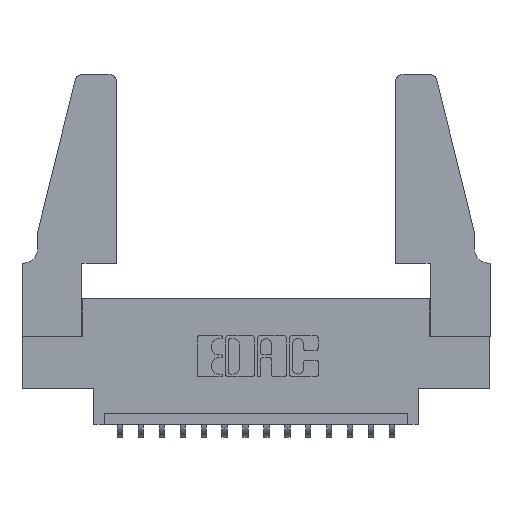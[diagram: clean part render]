
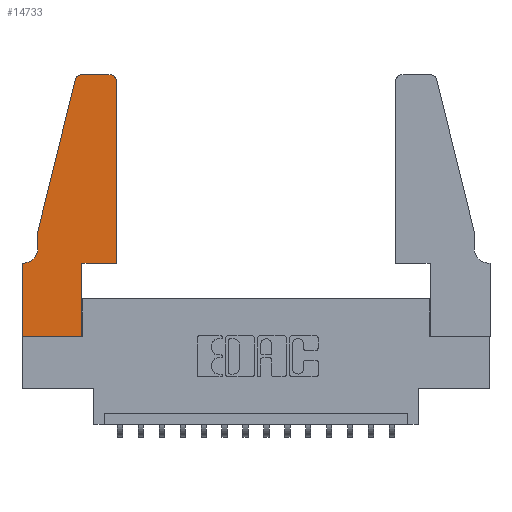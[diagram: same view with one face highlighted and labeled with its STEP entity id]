
A CAD part, top view. The second image highlights one B-rep face of the part: STEP entity #14733.
In plain terms, the highlighted planar face has unit normal (0, 0, 1).
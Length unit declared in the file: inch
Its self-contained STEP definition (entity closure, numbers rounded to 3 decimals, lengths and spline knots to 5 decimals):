
#76 = DIRECTION ( 'NONE',  ( 1., 0., 0. ) ) ;
#94 = CARTESIAN_POINT ( 'NONE',  ( 0.284, 1.25, 0.37 ) ) ;
#115 = AXIS2_PLACEMENT_3D ( 'NONE', #10868, #9346, #8216 ) ;
#148 = DIRECTION ( 'NONE',  ( 1., 0., 0. ) ) ;
#444 = VECTOR ( 'NONE', #148, 39.37008 ) ;
#656 = VECTOR ( 'NONE', #3718, 39.37008 ) ;
#695 = PLANE ( 'NONE',  #3113 ) ;
#698 = LINE ( 'NONE', #9634, #4725 ) ;
#718 = DIRECTION ( 'NONE',  ( 0., -1., 0. ) ) ;
#967 = AXIS2_PLACEMENT_3D ( 'NONE', #3220, #9567, #7124 ) ;
#976 = LINE ( 'NONE', #12297, #14297 ) ;
#1008 = VERTEX_POINT ( 'NONE', #6383 ) ;
#1136 = EDGE_LOOP ( 'NONE', ( #13993, #15913, #9920, #2115, #15725, #8309, #8147, #14769, #15879, #13197, #11582, #14621 ) ) ;
#1355 = DIRECTION ( 'NONE',  ( 0., 0., 1. ) ) ;
#1687 = LINE ( 'NONE', #6221, #16185 ) ;
#1898 = CIRCLE ( 'NONE', #967, 0.03 ) ;
#2115 = ORIENTED_EDGE ( 'NONE', *, *, #6302, .T. ) ;
#2418 = DIRECTION ( 'NONE',  ( 0., -1., 0. ) ) ;
#2438 = CARTESIAN_POINT ( 'NONE',  ( 0.0755, 0.35, 0.37 ) ) ;
#3079 = LINE ( 'NONE', #16092, #9703 ) ;
#3113 = AXIS2_PLACEMENT_3D ( 'NONE', #16163, #10983, #14784 ) ;
#3220 = CARTESIAN_POINT ( 'NONE',  ( 0.4205, 1.22, 0.37 ) ) ;
#3603 = VERTEX_POINT ( 'NONE', #14075 ) ;
#3718 = DIRECTION ( 'NONE',  ( 0., 1., 0. ) ) ;
#4295 = DIRECTION ( 'NONE',  ( 1., 0., 0. ) ) ;
#4384 = EDGE_CURVE ( 'NONE', #14108, #9184, #15170, .T. ) ;
#4507 = CARTESIAN_POINT ( 'NONE',  ( 0.0755, 0.5, 0.37 ) ) ;
#4725 = VECTOR ( 'NONE', #4295, 39.37008 ) ;
#4752 = CARTESIAN_POINT ( 'NONE',  ( 0.0755, 0.5, 0.37 ) ) ;
#4783 = DIRECTION ( 'NONE',  ( -1., 0., 0. ) ) ;
#4927 = CARTESIAN_POINT ( 'NONE',  ( 0.4205, 1.25, 0.37 ) ) ;
#5158 = DIRECTION ( 'NONE',  ( 0., 1., 0. ) ) ;
#5824 = CIRCLE ( 'NONE', #13679, 0.03 ) ;
#6013 = EDGE_CURVE ( 'NONE', #10647, #8459, #5824, .T. ) ;
#6221 = CARTESIAN_POINT ( 'NONE',  ( 0.4505, 0.35, 0.37 ) ) ;
#6302 = EDGE_CURVE ( 'NONE', #6446, #16093, #976, .T. ) ;
#6353 = CARTESIAN_POINT ( 'NONE',  ( 0.2605, 1.25, 0.37 ) ) ;
#6383 = CARTESIAN_POINT ( 'NONE',  ( 0.4505, 1.22, 0.37 ) ) ;
#6446 = VERTEX_POINT ( 'NONE', #4507 ) ;
#7049 = CIRCLE ( 'NONE', #115, 0.07 ) ;
#7124 = DIRECTION ( 'NONE',  ( 1., 0., 0. ) ) ;
#7454 = LINE ( 'NONE', #15557, #444 ) ;
#7640 = DIRECTION ( 'NONE',  ( -1., 0., 0. ) ) ;
#7692 = LINE ( 'NONE', #4752, #7885 ) ;
#7705 = CARTESIAN_POINT ( 'NONE',  ( 0.284, 1.22, 0.37 ) ) ;
#7885 = VECTOR ( 'NONE', #9975, 39.37008 ) ;
#8147 = ORIENTED_EDGE ( 'NONE', *, *, #14556, .T. ) ;
#8216 = DIRECTION ( 'NONE',  ( -1., 0., 0. ) ) ;
#8309 = ORIENTED_EDGE ( 'NONE', *, *, #4384, .T. ) ;
#8459 = VERTEX_POINT ( 'NONE', #15761 ) ;
#9184 = VERTEX_POINT ( 'NONE', #14046 ) ;
#9313 = VERTEX_POINT ( 'NONE', #12791 ) ;
#9346 = DIRECTION ( 'NONE',  ( 0., 0., -1. ) ) ;
#9567 = DIRECTION ( 'NONE',  ( 0., 0., 1. ) ) ;
#9588 = EDGE_CURVE ( 'NONE', #1008, #15036, #1898, .T. ) ;
#9634 = CARTESIAN_POINT ( 'NONE',  ( 0., 0., 0.37 ) ) ;
#9703 = VECTOR ( 'NONE', #2418, 39.37008 ) ;
#9885 = EDGE_CURVE ( 'NONE', #9940, #1008, #1687, .T. ) ;
#9920 = ORIENTED_EDGE ( 'NONE', *, *, #10413, .T. ) ;
#9940 = VERTEX_POINT ( 'NONE', #15263 ) ;
#9975 = DIRECTION ( 'NONE',  ( -0.239, -0.971, 0. ) ) ;
#10413 = EDGE_CURVE ( 'NONE', #8459, #6446, #7692, .T. ) ;
#10564 = VERTEX_POINT ( 'NONE', #15352 ) ;
#10647 = VERTEX_POINT ( 'NONE', #94 ) ;
#10868 = CARTESIAN_POINT ( 'NONE',  ( 0.0055, 0.42, 0.37 ) ) ;
#10983 = DIRECTION ( 'NONE',  ( 0., 0., 1. ) ) ;
#11087 = LINE ( 'NONE', #6353, #12283 ) ;
#11582 = ORIENTED_EDGE ( 'NONE', *, *, #9885, .T. ) ;
#12283 = VECTOR ( 'NONE', #7640, 39.37008 ) ;
#12297 = CARTESIAN_POINT ( 'NONE',  ( 0.0755, 0.5, 0.37 ) ) ;
#12791 = CARTESIAN_POINT ( 'NONE',  ( 0., 0., 0.37 ) ) ;
#13197 = ORIENTED_EDGE ( 'NONE', *, *, #15731, .T. ) ;
#13210 = EDGE_CURVE ( 'NONE', #9313, #10564, #698, .T. ) ;
#13679 = AXIS2_PLACEMENT_3D ( 'NONE', #7705, #1355, #76 ) ;
#13993 = ORIENTED_EDGE ( 'NONE', *, *, #16182, .T. ) ;
#14033 = CARTESIAN_POINT ( 'NONE',  ( 0.0755, 0.42, 0.37 ) ) ;
#14046 = CARTESIAN_POINT ( 'NONE',  ( 0., 0.35, 0.37 ) ) ;
#14075 = CARTESIAN_POINT ( 'NONE',  ( 0.2865, 0.35, 0.37 ) ) ;
#14108 = VERTEX_POINT ( 'NONE', #14530 ) ;
#14297 = VECTOR ( 'NONE', #718, 39.37008 ) ;
#14354 = EDGE_CURVE ( 'NONE', #10564, #3603, #14368, .T. ) ;
#14368 = LINE ( 'NONE', #15276, #656 ) ;
#14530 = CARTESIAN_POINT ( 'NONE',  ( 0.0055, 0.35, 0.37 ) ) ;
#14556 = EDGE_CURVE ( 'NONE', #9184, #9313, #3079, .T. ) ;
#14621 = ORIENTED_EDGE ( 'NONE', *, *, #9588, .T. ) ;
#14733 = ADVANCED_FACE ( 'NONE', ( #15544 ), #695, .T. ) ;
#14769 = ORIENTED_EDGE ( 'NONE', *, *, #13210, .T. ) ;
#14784 = DIRECTION ( 'NONE',  ( 1., 0., 0. ) ) ;
#15036 = VERTEX_POINT ( 'NONE', #4927 ) ;
#15170 = LINE ( 'NONE', #2438, #16159 ) ;
#15263 = CARTESIAN_POINT ( 'NONE',  ( 0.4505, 0.35, 0.37 ) ) ;
#15276 = CARTESIAN_POINT ( 'NONE',  ( 0.2865, 0.35, 0.37 ) ) ;
#15352 = CARTESIAN_POINT ( 'NONE',  ( 0.2865, 0., 0.37 ) ) ;
#15544 = FACE_OUTER_BOUND ( 'NONE', #1136, .T. ) ;
#15557 = CARTESIAN_POINT ( 'NONE',  ( 0.4505, 0.35, 0.37 ) ) ;
#15725 = ORIENTED_EDGE ( 'NONE', *, *, #15872, .T. ) ;
#15731 = EDGE_CURVE ( 'NONE', #3603, #9940, #7454, .T. ) ;
#15761 = CARTESIAN_POINT ( 'NONE',  ( 0.25487, 1.22718, 0.37 ) ) ;
#15872 = EDGE_CURVE ( 'NONE', #16093, #14108, #7049, .T. ) ;
#15879 = ORIENTED_EDGE ( 'NONE', *, *, #14354, .T. ) ;
#15913 = ORIENTED_EDGE ( 'NONE', *, *, #6013, .T. ) ;
#16092 = CARTESIAN_POINT ( 'NONE',  ( 0., 0., 0.37 ) ) ;
#16093 = VERTEX_POINT ( 'NONE', #14033 ) ;
#16159 = VECTOR ( 'NONE', #4783, 39.37008 ) ;
#16163 = CARTESIAN_POINT ( 'NONE',  ( 0., 0.35, 0.37 ) ) ;
#16182 = EDGE_CURVE ( 'NONE', #15036, #10647, #11087, .T. ) ;
#16185 = VECTOR ( 'NONE', #5158, 39.37008 ) ;
